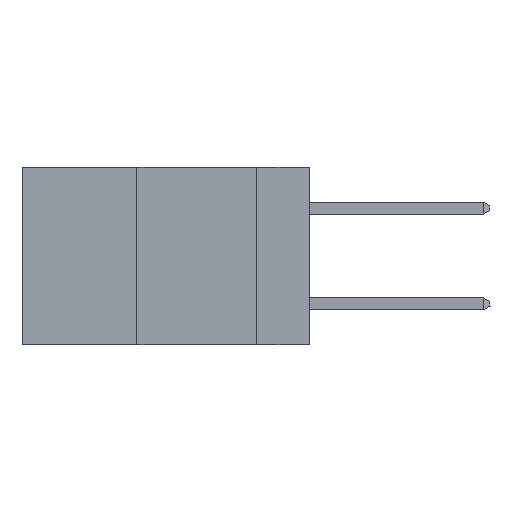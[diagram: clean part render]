
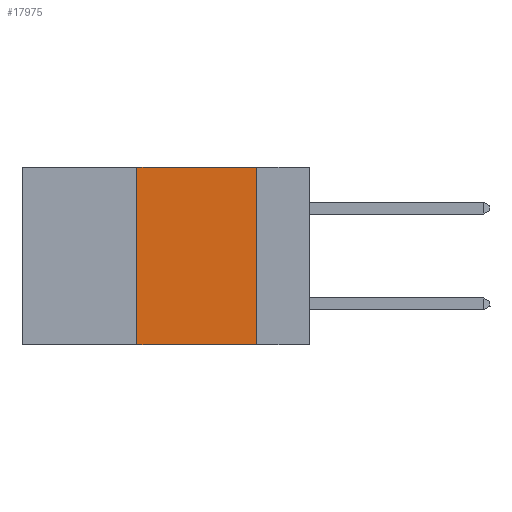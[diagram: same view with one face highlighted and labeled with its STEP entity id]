
A CAD part, left-side view. The second image highlights one B-rep face of the part: STEP entity #17975.
In plain terms, the highlighted planar face has unit normal (-1, 0, 0).
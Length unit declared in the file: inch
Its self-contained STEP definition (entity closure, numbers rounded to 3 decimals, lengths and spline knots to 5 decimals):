
#1699 = VECTOR ( 'NONE', #24607, 39.37008 ) ;
#3967 = DIRECTION ( 'NONE',  ( 0., 0., -1. ) ) ;
#6403 = CARTESIAN_POINT ( 'NONE',  ( 0., 0.36, 0. ) ) ;
#6847 = EDGE_CURVE ( 'NONE', #24837, #16323, #10309, .T. ) ;
#7018 = VECTOR ( 'NONE', #15307, 39.37008 ) ;
#8637 = EDGE_CURVE ( 'NONE', #18101, #9078, #24913, .T. ) ;
#9078 = VERTEX_POINT ( 'NONE', #15098 ) ;
#9620 = CARTESIAN_POINT ( 'NONE',  ( 0., 0.11, 0. ) ) ;
#10309 = LINE ( 'NONE', #13709, #1699 ) ;
#13709 = CARTESIAN_POINT ( 'NONE',  ( 0., 0.11, 0. ) ) ;
#13776 = DIRECTION ( 'NONE',  ( 0., -1., 0. ) ) ;
#14141 = ORIENTED_EDGE ( 'NONE', *, *, #8637, .F. ) ;
#15098 = CARTESIAN_POINT ( 'NONE',  ( 0., 0.36, 0. ) ) ;
#15307 = DIRECTION ( 'NONE',  ( 0., -1., 0. ) ) ;
#15514 = EDGE_CURVE ( 'NONE', #18101, #16323, #19112, .T. ) ;
#16323 = VERTEX_POINT ( 'NONE', #27761 ) ;
#17559 = VECTOR ( 'NONE', #25504, 39.37008 ) ;
#17975 = ADVANCED_FACE ( 'NONE', ( #35428 ), #31499, .F. ) ;
#18101 = VERTEX_POINT ( 'NONE', #24154 ) ;
#18903 = ORIENTED_EDGE ( 'NONE', *, *, #15514, .T. ) ;
#19112 = LINE ( 'NONE', #31591, #7018 ) ;
#19264 = AXIS2_PLACEMENT_3D ( 'NONE', #34261, #20540, #3967 ) ;
#19852 = ORIENTED_EDGE ( 'NONE', *, *, #23390, .F. ) ;
#20540 = DIRECTION ( 'NONE',  ( 1., 0., 0. ) ) ;
#23390 = EDGE_CURVE ( 'NONE', #9078, #24837, #30544, .T. ) ;
#24154 = CARTESIAN_POINT ( 'NONE',  ( 0., 0.36, -0.37 ) ) ;
#24607 = DIRECTION ( 'NONE',  ( 0., 0., -1. ) ) ;
#24837 = VERTEX_POINT ( 'NONE', #9620 ) ;
#24913 = LINE ( 'NONE', #6403, #17559 ) ;
#25504 = DIRECTION ( 'NONE',  ( 0., 0., 1. ) ) ;
#27761 = CARTESIAN_POINT ( 'NONE',  ( 0., 0.11, -0.37 ) ) ;
#28827 = VECTOR ( 'NONE', #13776, 39.37008 ) ;
#29427 = EDGE_LOOP ( 'NONE', ( #34837, #19852, #14141, #18903 ) ) ;
#30362 = CARTESIAN_POINT ( 'NONE',  ( 0., 0.6, 0. ) ) ;
#30544 = LINE ( 'NONE', #30362, #28827 ) ;
#31499 = PLANE ( 'NONE',  #19264 ) ;
#31591 = CARTESIAN_POINT ( 'NONE',  ( 0., 0.6, -0.37 ) ) ;
#34261 = CARTESIAN_POINT ( 'NONE',  ( 0., 0.6, 0. ) ) ;
#34837 = ORIENTED_EDGE ( 'NONE', *, *, #6847, .F. ) ;
#35428 = FACE_OUTER_BOUND ( 'NONE', #29427, .T. ) ;
